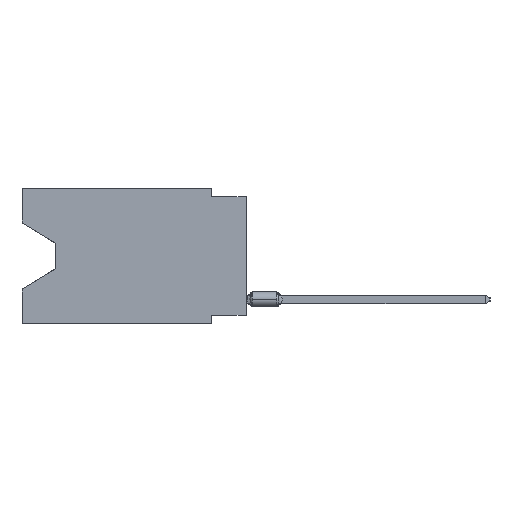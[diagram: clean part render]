
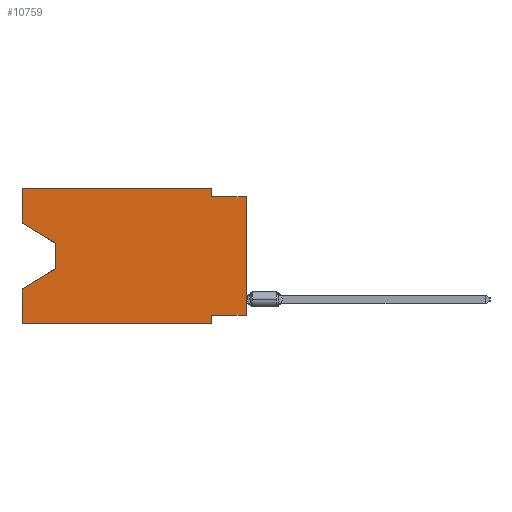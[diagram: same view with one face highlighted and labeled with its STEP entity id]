
A CAD part, left-side view. The second image highlights one B-rep face of the part: STEP entity #10759.
In plain terms, the highlighted planar face has unit normal (-1, 0, 0).
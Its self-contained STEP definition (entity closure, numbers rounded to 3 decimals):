
#333 = AXIS2_PLACEMENT_3D ( 'NONE', #23240, #20696, #29898 ) ;
#352 = EDGE_CURVE ( 'NONE', #36696, #32436, #2786, .T. ) ;
#412 = LINE ( 'NONE', #18528, #1074 ) ;
#938 = VECTOR ( 'NONE', #34032, 1000. ) ;
#1074 = VECTOR ( 'NONE', #6322, 1000. ) ;
#1660 = EDGE_CURVE ( 'NONE', #38697, #37865, #21570, .T. ) ;
#2192 = FACE_OUTER_BOUND ( 'NONE', #37273, .T. ) ;
#2266 = CARTESIAN_POINT ( 'NONE',  ( 0., 16.383, 0. ) ) ;
#2461 = DIRECTION ( 'NONE',  ( 0., 0., -1. ) ) ;
#2653 = CARTESIAN_POINT ( 'NONE',  ( 0., 13.97, -4.013 ) ) ;
#2762 = ORIENTED_EDGE ( 'NONE', *, *, #14169, .F. ) ;
#2786 = LINE ( 'NONE', #5349, #14908 ) ;
#2861 = VECTOR ( 'NONE', #17538, 1000. ) ;
#2960 = LINE ( 'NONE', #18288, #14354 ) ;
#3207 = VERTEX_POINT ( 'NONE', #2266 ) ;
#3228 = EDGE_CURVE ( 'NONE', #8238, #36696, #20383, .T. ) ;
#4812 = DIRECTION ( 'NONE',  ( 0., -0.855, -0.519 ) ) ;
#5232 = VECTOR ( 'NONE', #4812, 1000. ) ;
#5349 = CARTESIAN_POINT ( 'NONE',  ( 0., 13.97, -5.893 ) ) ;
#5568 = EDGE_CURVE ( 'NONE', #38697, #8391, #9374, .T. ) ;
#5731 = VERTEX_POINT ( 'NONE', #25482 ) ;
#6256 = DIRECTION ( 'NONE',  ( 0., -1., 0. ) ) ;
#6322 = DIRECTION ( 'NONE',  ( 0., 0., 1. ) ) ;
#6609 = DIRECTION ( 'NONE',  ( 0., 0., 1. ) ) ;
#6912 = ORIENTED_EDGE ( 'NONE', *, *, #1660, .F. ) ;
#7952 = ORIENTED_EDGE ( 'NONE', *, *, #26958, .T. ) ;
#8151 = VERTEX_POINT ( 'NONE', #15156 ) ;
#8238 = VERTEX_POINT ( 'NONE', #31050 ) ;
#8391 = VERTEX_POINT ( 'NONE', #13763 ) ;
#8504 = CARTESIAN_POINT ( 'NONE',  ( 0., 16.383, 0. ) ) ;
#9085 = EDGE_CURVE ( 'NONE', #37865, #35265, #22086, .T. ) ;
#9243 = EDGE_CURVE ( 'NONE', #18546, #32436, #35774, .T. ) ;
#9374 = LINE ( 'NONE', #32943, #30337 ) ;
#9830 = LINE ( 'NONE', #33964, #22978 ) ;
#10117 = LINE ( 'NONE', #33165, #29772 ) ;
#10236 = EDGE_CURVE ( 'NONE', #3207, #8151, #10117, .T. ) ;
#10759 = ADVANCED_FACE ( 'NONE', ( #2192 ), #11253, .F. ) ;
#10974 = ORIENTED_EDGE ( 'NONE', *, *, #10236, .F. ) ;
#11253 = PLANE ( 'NONE',  #333 ) ;
#11530 = ORIENTED_EDGE ( 'NONE', *, *, #9243, .F. ) ;
#12321 = CARTESIAN_POINT ( 'NONE',  ( 0., 0., -9.271 ) ) ;
#12689 = ORIENTED_EDGE ( 'NONE', *, *, #15032, .F. ) ;
#13763 = CARTESIAN_POINT ( 'NONE',  ( 0., 0., -0.635 ) ) ;
#13789 = CARTESIAN_POINT ( 'NONE',  ( 0., 2.54, -9.906 ) ) ;
#14169 = EDGE_CURVE ( 'NONE', #5731, #8391, #9830, .T. ) ;
#14354 = VECTOR ( 'NONE', #38485, 1000. ) ;
#14908 = VECTOR ( 'NONE', #15159, 1000. ) ;
#15032 = EDGE_CURVE ( 'NONE', #29754, #3207, #412, .T. ) ;
#15156 = CARTESIAN_POINT ( 'NONE',  ( 0., 2.54, 0. ) ) ;
#15159 = DIRECTION ( 'NONE',  ( 0., 0.855, -0.519 ) ) ;
#16732 = CARTESIAN_POINT ( 'NONE',  ( 0., 2.54, -9.271 ) ) ;
#17532 = ORIENTED_EDGE ( 'NONE', *, *, #5568, .T. ) ;
#17538 = DIRECTION ( 'NONE',  ( 0., 0., 1. ) ) ;
#18288 = CARTESIAN_POINT ( 'NONE',  ( 0., 2.54, 0. ) ) ;
#18528 = CARTESIAN_POINT ( 'NONE',  ( 0., 16.383, 0. ) ) ;
#18546 = VERTEX_POINT ( 'NONE', #29246 ) ;
#19184 = ORIENTED_EDGE ( 'NONE', *, *, #21969, .F. ) ;
#19272 = DIRECTION ( 'NONE',  ( 0., -1., 0. ) ) ;
#20383 = LINE ( 'NONE', #2653, #32004 ) ;
#20696 = DIRECTION ( 'NONE',  ( 1., 0., 0. ) ) ;
#20944 = EDGE_CURVE ( 'NONE', #18546, #35265, #22939, .T. ) ;
#21570 = LINE ( 'NONE', #12321, #33681 ) ;
#21769 = DIRECTION ( 'NONE',  ( 0., 1., 0. ) ) ;
#21969 = EDGE_CURVE ( 'NONE', #8151, #5731, #2960, .T. ) ;
#22086 = LINE ( 'NONE', #28164, #938 ) ;
#22939 = LINE ( 'NONE', #29586, #32476 ) ;
#22978 = VECTOR ( 'NONE', #19272, 1000. ) ;
#23240 = CARTESIAN_POINT ( 'NONE',  ( 0., 16.383, 0. ) ) ;
#23525 = DIRECTION ( 'NONE',  ( 0., -1., 0. ) ) ;
#24677 = CARTESIAN_POINT ( 'NONE',  ( 0., 16.383, -2.546 ) ) ;
#25482 = CARTESIAN_POINT ( 'NONE',  ( 0., 2.54, -0.635 ) ) ;
#26744 = ORIENTED_EDGE ( 'NONE', *, *, #3228, .T. ) ;
#26958 = EDGE_CURVE ( 'NONE', #29754, #8238, #35445, .T. ) ;
#27700 = CARTESIAN_POINT ( 'NONE',  ( 0., 13.97, -5.893 ) ) ;
#28164 = CARTESIAN_POINT ( 'NONE',  ( 0., 2.54, -9.906 ) ) ;
#29246 = CARTESIAN_POINT ( 'NONE',  ( 0., 16.383, -9.906 ) ) ;
#29586 = CARTESIAN_POINT ( 'NONE',  ( 0., 16.383, -9.906 ) ) ;
#29754 = VERTEX_POINT ( 'NONE', #24677 ) ;
#29772 = VECTOR ( 'NONE', #6256, 1000. ) ;
#29898 = DIRECTION ( 'NONE',  ( 0., 0., -1. ) ) ;
#29911 = ORIENTED_EDGE ( 'NONE', *, *, #352, .T. ) ;
#30337 = VECTOR ( 'NONE', #6609, 1000. ) ;
#31050 = CARTESIAN_POINT ( 'NONE',  ( 0., 13.97, -4.013 ) ) ;
#31867 = CARTESIAN_POINT ( 'NONE',  ( 0., 0., -9.271 ) ) ;
#31926 = CARTESIAN_POINT ( 'NONE',  ( 0., 16.383, -2.546 ) ) ;
#32004 = VECTOR ( 'NONE', #2461, 1000. ) ;
#32436 = VERTEX_POINT ( 'NONE', #38219 ) ;
#32476 = VECTOR ( 'NONE', #23525, 1000. ) ;
#32943 = CARTESIAN_POINT ( 'NONE',  ( 0., 0., 0. ) ) ;
#33165 = CARTESIAN_POINT ( 'NONE',  ( 0., 16.383, 0. ) ) ;
#33392 = ORIENTED_EDGE ( 'NONE', *, *, #20944, .T. ) ;
#33681 = VECTOR ( 'NONE', #21769, 1000. ) ;
#33964 = CARTESIAN_POINT ( 'NONE',  ( 0., 0., -0.635 ) ) ;
#34032 = DIRECTION ( 'NONE',  ( 0., 0., -1. ) ) ;
#35265 = VERTEX_POINT ( 'NONE', #13789 ) ;
#35445 = LINE ( 'NONE', #31926, #5232 ) ;
#35774 = LINE ( 'NONE', #8504, #2861 ) ;
#36696 = VERTEX_POINT ( 'NONE', #27700 ) ;
#36898 = ORIENTED_EDGE ( 'NONE', *, *, #9085, .F. ) ;
#37273 = EDGE_LOOP ( 'NONE', ( #7952, #26744, #29911, #11530, #33392, #36898, #6912, #17532, #2762, #19184, #10974, #12689 ) ) ;
#37865 = VERTEX_POINT ( 'NONE', #16732 ) ;
#38219 = CARTESIAN_POINT ( 'NONE',  ( 0., 16.383, -7.36 ) ) ;
#38485 = DIRECTION ( 'NONE',  ( 0., 0., -1. ) ) ;
#38697 = VERTEX_POINT ( 'NONE', #31867 ) ;
